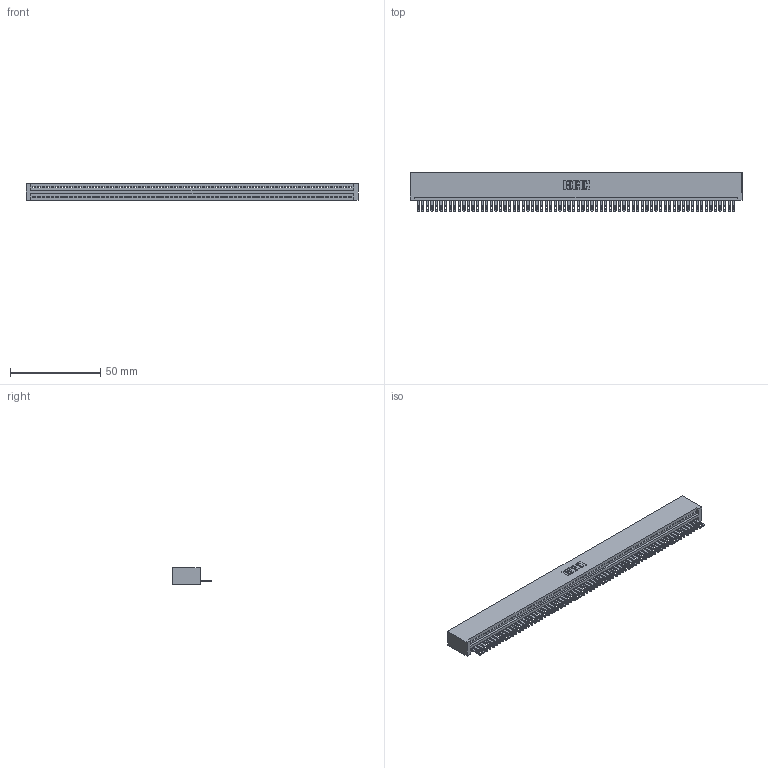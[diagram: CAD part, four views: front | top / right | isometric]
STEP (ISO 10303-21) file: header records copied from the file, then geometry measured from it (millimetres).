
FILE_DESCRIPTION (( 'STEP AP203' ), '1' );
FILE_NAME ('345-070-500-101.STEP', '2018-09-30T21:13:58', ( '' ), ( '' ), 'SwSTEP 2.0', 'SolidWorks 2016', '' );
FILE_SCHEMA (( 'CONFIG_CONTROL_DESIGN' ));
Length unit declared in the file: inch
Products named in the file (3): 345-292-001_345-293-100; 345-070-500-101; 345 Part_No Mounting Lugs
Assembly tree (71 placements, depth 2):
  345-070-500-101
    345 Part_No Mounting Lugs
    345-292-001_345-293-100  x70
Bounding box: 184.4 x 21.51 x 9.4 mm (x, y, z)
Volume: 18371.9 mm3; surface area: 25142.5 mm2
Topology: 71 solids, 71 shells, 3898 faces, 12077 edges, 8050 vertices
Faces by surface type: plane 2456, cylinder 1442
Entity records: 48567 total; most frequent: ORIENTED_EDGE 8422, CARTESIAN_POINT 8418, DIRECTION 7307, EDGE_CURVE 4211, LINE 3803, VECTOR 3803, VERTEX_POINT 2806, AXIS2_PLACEMENT_3D 1752
